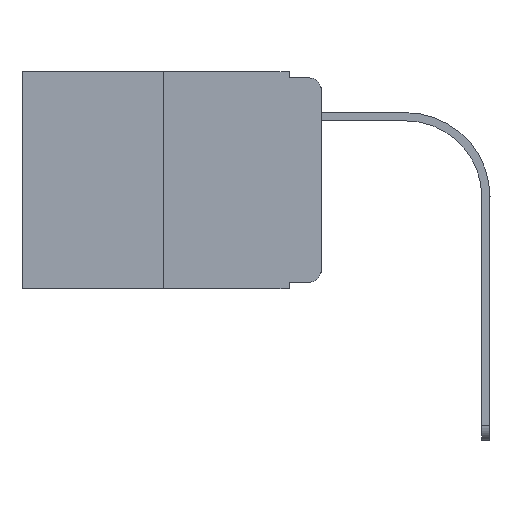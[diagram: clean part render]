
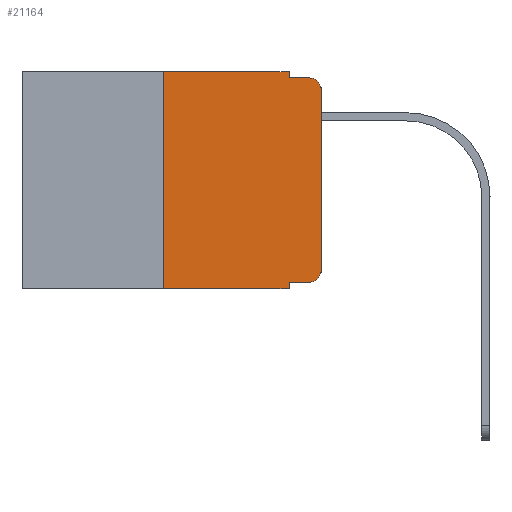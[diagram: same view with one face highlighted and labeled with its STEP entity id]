
A CAD part, left-side view. The second image highlights one B-rep face of the part: STEP entity #21164.
In plain terms, the highlighted planar face has unit normal (-1, 0, 0).
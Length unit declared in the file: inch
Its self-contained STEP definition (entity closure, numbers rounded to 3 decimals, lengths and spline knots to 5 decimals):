
#264 = VERTEX_POINT ( 'NONE', #15103 ) ;
#329 = VECTOR ( 'NONE', #14361, 39.37008 ) ;
#1257 = EDGE_CURVE ( 'NONE', #17831, #5735, #24165, .T. ) ;
#1284 = ORIENTED_EDGE ( 'NONE', *, *, #12740, .T. ) ;
#1311 = ORIENTED_EDGE ( 'NONE', *, *, #4192, .T. ) ;
#1730 = CARTESIAN_POINT ( 'NONE',  ( 0., 0., 0. ) ) ;
#1851 = CARTESIAN_POINT ( 'NONE',  ( 0., 0., -0.313 ) ) ;
#1969 = CARTESIAN_POINT ( 'NONE',  ( 0., 0., -0.03 ) ) ;
#2040 = EDGE_CURVE ( 'NONE', #10973, #10090, #18607, .T. ) ;
#2445 = EDGE_CURVE ( 'NONE', #5735, #14584, #14521, .T. ) ;
#2459 = DIRECTION ( 'NONE',  ( 0., 0., -1. ) ) ;
#3017 = EDGE_CURVE ( 'NONE', #8902, #5642, #25051, .T. ) ;
#3352 = CARTESIAN_POINT ( 'NONE',  ( 0., 0.051, -0.01 ) ) ;
#3422 = DIRECTION ( 'NONE',  ( -1., 0., 0. ) ) ;
#3734 = ORIENTED_EDGE ( 'NONE', *, *, #3017, .T. ) ;
#4078 = VECTOR ( 'NONE', #10728, 39.37008 ) ;
#4192 = EDGE_CURVE ( 'NONE', #10973, #8902, #19895, .T. ) ;
#5003 = CARTESIAN_POINT ( 'NONE',  ( 0., 0.051, 0. ) ) ;
#5122 = VECTOR ( 'NONE', #7972, 39.37008 ) ;
#5165 = DIRECTION ( 'NONE',  ( 0., 0., -1. ) ) ;
#5519 = VECTOR ( 'NONE', #24254, 39.37008 ) ;
#5642 = VERTEX_POINT ( 'NONE', #1851 ) ;
#5690 = DIRECTION ( 'NONE',  ( 0., -1., 0. ) ) ;
#5735 = VERTEX_POINT ( 'NONE', #17736 ) ;
#6758 = CARTESIAN_POINT ( 'NONE',  ( 0., 0.473, -0.343 ) ) ;
#7520 = VECTOR ( 'NONE', #5690, 39.37008 ) ;
#7553 = CARTESIAN_POINT ( 'NONE',  ( 0., 0.473, 0. ) ) ;
#7598 = LINE ( 'NONE', #23114, #7520 ) ;
#7972 = DIRECTION ( 'NONE',  ( 0., 0., 1. ) ) ;
#8476 = VECTOR ( 'NONE', #2459, 39.37008 ) ;
#8666 = CARTESIAN_POINT ( 'NONE',  ( 0., 0.25, 0. ) ) ;
#8902 = VERTEX_POINT ( 'NONE', #19993 ) ;
#9026 = VECTOR ( 'NONE', #12224, 39.37008 ) ;
#9206 = VERTEX_POINT ( 'NONE', #1969 ) ;
#9636 = AXIS2_PLACEMENT_3D ( 'NONE', #14992, #3422, #16750 ) ;
#9718 = EDGE_CURVE ( 'NONE', #15488, #17831, #16495, .T. ) ;
#10090 = VERTEX_POINT ( 'NONE', #19995 ) ;
#10728 = DIRECTION ( 'NONE',  ( 0., 0., -1. ) ) ;
#10893 = EDGE_CURVE ( 'NONE', #15488, #10090, #21746, .T. ) ;
#10973 = VERTEX_POINT ( 'NONE', #12332 ) ;
#11491 = DIRECTION ( 'NONE',  ( 1., 0., 0. ) ) ;
#11624 = FACE_OUTER_BOUND ( 'NONE', #24670, .T. ) ;
#12169 = DIRECTION ( 'NONE',  ( 0., -1., 0. ) ) ;
#12224 = DIRECTION ( 'NONE',  ( 0., -1., 0. ) ) ;
#12332 = CARTESIAN_POINT ( 'NONE',  ( 0., 0.051, -0.333 ) ) ;
#12740 = EDGE_CURVE ( 'NONE', #9206, #264, #13314, .T. ) ;
#13314 = CIRCLE ( 'NONE', #14122, 0.02 ) ;
#14122 = AXIS2_PLACEMENT_3D ( 'NONE', #15063, #20650, #5165 ) ;
#14255 = CARTESIAN_POINT ( 'NONE',  ( 0., 0.473, 0. ) ) ;
#14332 = CARTESIAN_POINT ( 'NONE',  ( 0., 0.25, 0. ) ) ;
#14361 = DIRECTION ( 'NONE',  ( 0., -1., 0. ) ) ;
#14521 = LINE ( 'NONE', #18317, #8476 ) ;
#14584 = VERTEX_POINT ( 'NONE', #3352 ) ;
#14634 = ORIENTED_EDGE ( 'NONE', *, *, #2040, .F. ) ;
#14794 = ORIENTED_EDGE ( 'NONE', *, *, #20225, .T. ) ;
#14992 = CARTESIAN_POINT ( 'NONE',  ( 0., 0.02, -0.313 ) ) ;
#15063 = CARTESIAN_POINT ( 'NONE',  ( 0., 0.02, -0.03 ) ) ;
#15103 = CARTESIAN_POINT ( 'NONE',  ( 0., 0.02, -0.01 ) ) ;
#15314 = DIRECTION ( 'NONE',  ( 0., 0., -1. ) ) ;
#15488 = VERTEX_POINT ( 'NONE', #19283 ) ;
#15590 = AXIS2_PLACEMENT_3D ( 'NONE', #7553, #11491, #15314 ) ;
#15669 = ORIENTED_EDGE ( 'NONE', *, *, #2445, .F. ) ;
#16133 = ORIENTED_EDGE ( 'NONE', *, *, #23606, .F. ) ;
#16495 = LINE ( 'NONE', #14332, #5519 ) ;
#16750 = DIRECTION ( 'NONE',  ( 0., 0., -1. ) ) ;
#17370 = LINE ( 'NONE', #1730, #5122 ) ;
#17736 = CARTESIAN_POINT ( 'NONE',  ( 0., 0.051, 0. ) ) ;
#17831 = VERTEX_POINT ( 'NONE', #8666 ) ;
#18317 = CARTESIAN_POINT ( 'NONE',  ( 0., 0.051, 0. ) ) ;
#18607 = LINE ( 'NONE', #5003, #4078 ) ;
#18880 = ORIENTED_EDGE ( 'NONE', *, *, #10893, .T. ) ;
#19283 = CARTESIAN_POINT ( 'NONE',  ( 0., 0.25, -0.343 ) ) ;
#19895 = LINE ( 'NONE', #21444, #22532 ) ;
#19993 = CARTESIAN_POINT ( 'NONE',  ( 0., 0.02, -0.333 ) ) ;
#19995 = CARTESIAN_POINT ( 'NONE',  ( 0., 0.051, -0.343 ) ) ;
#20225 = EDGE_CURVE ( 'NONE', #5642, #9206, #17370, .T. ) ;
#20650 = DIRECTION ( 'NONE',  ( -1., 0., 0. ) ) ;
#20744 = ORIENTED_EDGE ( 'NONE', *, *, #9718, .F. ) ;
#21164 = ADVANCED_FACE ( 'NONE', ( #11624 ), #24825, .F. ) ;
#21444 = CARTESIAN_POINT ( 'NONE',  ( 0., 0.051, -0.333 ) ) ;
#21746 = LINE ( 'NONE', #6758, #329 ) ;
#21918 = ORIENTED_EDGE ( 'NONE', *, *, #1257, .F. ) ;
#22532 = VECTOR ( 'NONE', #12169, 39.37008 ) ;
#23114 = CARTESIAN_POINT ( 'NONE',  ( 0., 0.051, -0.01 ) ) ;
#23606 = EDGE_CURVE ( 'NONE', #14584, #264, #7598, .T. ) ;
#24165 = LINE ( 'NONE', #14255, #9026 ) ;
#24254 = DIRECTION ( 'NONE',  ( 0., 0., 1. ) ) ;
#24670 = EDGE_LOOP ( 'NONE', ( #14794, #1284, #16133, #15669, #21918, #20744, #18880, #14634, #1311, #3734 ) ) ;
#24825 = PLANE ( 'NONE',  #15590 ) ;
#25051 = CIRCLE ( 'NONE', #9636, 0.02 ) ;
